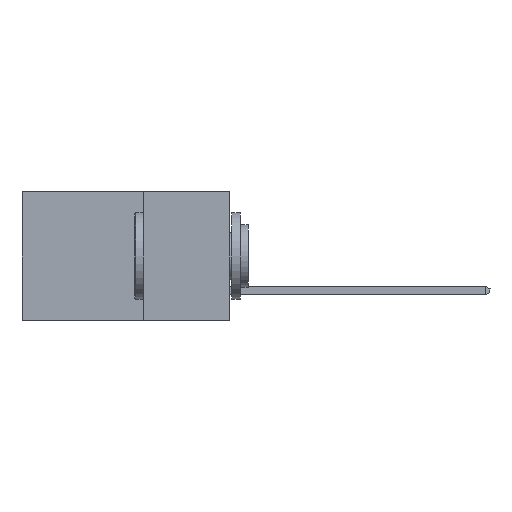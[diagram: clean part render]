
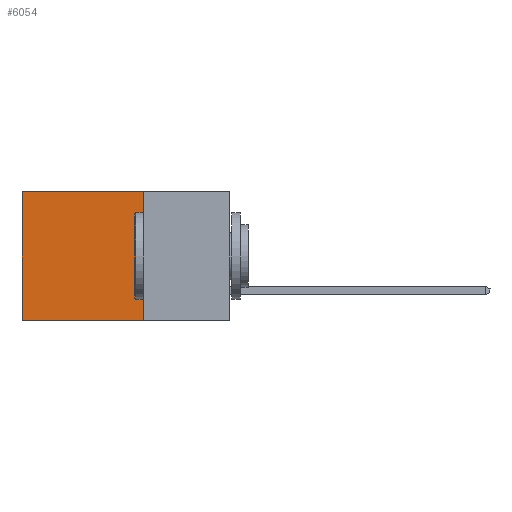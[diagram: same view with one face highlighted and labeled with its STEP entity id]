
A CAD part, left-side view. The second image highlights one B-rep face of the part: STEP entity #6054.
In plain terms, the highlighted planar face has unit normal (-1, 0, 0).
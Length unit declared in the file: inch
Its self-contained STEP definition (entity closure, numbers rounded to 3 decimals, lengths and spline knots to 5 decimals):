
#313 = EDGE_LOOP ( 'NONE', ( #1682, #6868, #9854, #7328 ) ) ;
#701 = VERTEX_POINT ( 'NONE', #10674 ) ;
#1682 = ORIENTED_EDGE ( 'NONE', *, *, #5488, .T. ) ;
#2270 = DIRECTION ( 'NONE',  ( 0., 0., -1. ) ) ;
#2297 = LINE ( 'NONE', #9353, #11153 ) ;
#2546 = VERTEX_POINT ( 'NONE', #4425 ) ;
#3537 = VERTEX_POINT ( 'NONE', #10945 ) ;
#4106 = DIRECTION ( 'NONE',  ( 0., 1., 0. ) ) ;
#4140 = FACE_OUTER_BOUND ( 'NONE', #313, .T. ) ;
#4425 = CARTESIAN_POINT ( 'NONE',  ( 0.2615, 0.6, -0.37 ) ) ;
#4884 = AXIS2_PLACEMENT_3D ( 'NONE', #7675, #6900, #11169 ) ;
#4913 = VERTEX_POINT ( 'NONE', #5924 ) ;
#5093 = LINE ( 'NONE', #9498, #6037 ) ;
#5488 = EDGE_CURVE ( 'NONE', #4913, #2546, #11330, .T. ) ;
#5905 = EDGE_CURVE ( 'NONE', #3537, #4913, #10142, .T. ) ;
#5924 = CARTESIAN_POINT ( 'NONE',  ( 0.2615, 0.6, 0. ) ) ;
#6037 = VECTOR ( 'NONE', #6710, 39.37008 ) ;
#6054 = ADVANCED_FACE ( 'NONE', ( #4140 ), #10252, .F. ) ;
#6673 = VECTOR ( 'NONE', #9977, 39.37008 ) ;
#6702 = VECTOR ( 'NONE', #2270, 39.37008 ) ;
#6710 = DIRECTION ( 'NONE',  ( 0., 0., -1. ) ) ;
#6868 = ORIENTED_EDGE ( 'NONE', *, *, #6898, .F. ) ;
#6898 = EDGE_CURVE ( 'NONE', #701, #2546, #2297, .T. ) ;
#6900 = DIRECTION ( 'NONE',  ( 1., 0., 0. ) ) ;
#7328 = ORIENTED_EDGE ( 'NONE', *, *, #5905, .T. ) ;
#7675 = CARTESIAN_POINT ( 'NONE',  ( 0.2615, 0.25, -0.37 ) ) ;
#7839 = EDGE_CURVE ( 'NONE', #3537, #701, #5093, .T. ) ;
#8192 = CARTESIAN_POINT ( 'NONE',  ( 0.2615, 0.25, 0. ) ) ;
#9353 = CARTESIAN_POINT ( 'NONE',  ( 0.2615, 0.25, -0.37 ) ) ;
#9498 = CARTESIAN_POINT ( 'NONE',  ( 0.2615, 0.25, -0.37 ) ) ;
#9854 = ORIENTED_EDGE ( 'NONE', *, *, #7839, .F. ) ;
#9977 = DIRECTION ( 'NONE',  ( 0., 1., 0. ) ) ;
#10142 = LINE ( 'NONE', #8192, #6673 ) ;
#10183 = CARTESIAN_POINT ( 'NONE',  ( 0.2615, 0.6, -0.37 ) ) ;
#10252 = PLANE ( 'NONE',  #4884 ) ;
#10674 = CARTESIAN_POINT ( 'NONE',  ( 0.2615, 0.25, -0.37 ) ) ;
#10945 = CARTESIAN_POINT ( 'NONE',  ( 0.2615, 0.25, 0. ) ) ;
#11153 = VECTOR ( 'NONE', #4106, 39.37008 ) ;
#11169 = DIRECTION ( 'NONE',  ( 0., 0., -1. ) ) ;
#11330 = LINE ( 'NONE', #10183, #6702 ) ;
